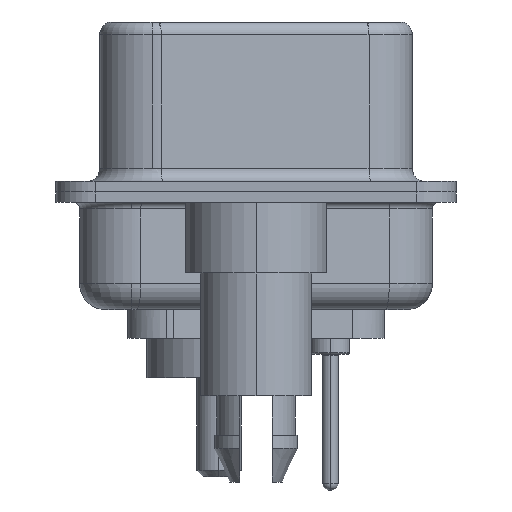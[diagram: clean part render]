
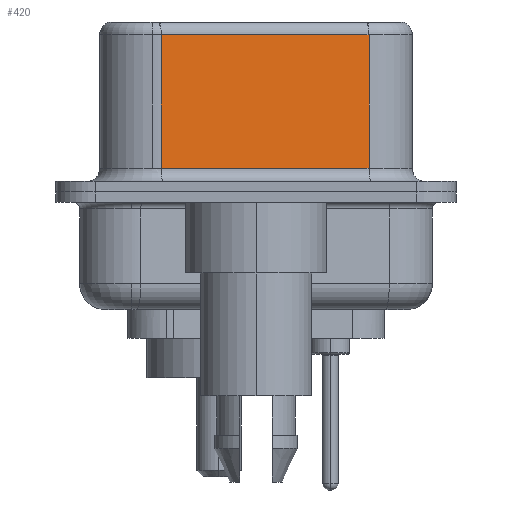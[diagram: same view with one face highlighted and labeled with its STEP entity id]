
A CAD part, left-side view. The second image highlights one B-rep face of the part: STEP entity #420.
In plain terms, the highlighted planar face has unit normal (-0.985, -0.174, 0).
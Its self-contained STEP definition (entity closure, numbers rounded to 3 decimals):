
#354 = PLANE ( 'NONE',  #21658 ) ;
#420 = ADVANCED_FACE ( 'NONE', ( #16871 ), #354, .F. ) ;
#1713 = VECTOR ( 'NONE', #21251, 1000. ) ;
#2260 = LINE ( 'NONE', #19577, #1713 ) ;
#2346 = VERTEX_POINT ( 'NONE', #6088 ) ;
#2419 = ORIENTED_EDGE ( 'NONE', *, *, #6296, .T. ) ;
#3163 = EDGE_LOOP ( 'NONE', ( #19923, #2419, #15302, #13762 ) ) ;
#3882 = DIRECTION ( 'NONE',  ( -0.174, 0.985, 0. ) ) ;
#4128 = CARTESIAN_POINT ( 'NONE',  ( 5.132, -4.322, 6.02 ) ) ;
#5108 = CARTESIAN_POINT ( 'NONE',  ( 5.132, -4.322, 6.52 ) ) ;
#5414 = EDGE_CURVE ( 'NONE', #2346, #11596, #9082, .T. ) ;
#5584 = CARTESIAN_POINT ( 'NONE',  ( 5.132, -4.322, 6.52 ) ) ;
#6088 = CARTESIAN_POINT ( 'NONE',  ( 3.73, 3.628, 6.02 ) ) ;
#6296 = EDGE_CURVE ( 'NONE', #20462, #2346, #14081, .T. ) ;
#6843 = DIRECTION ( 'NONE',  ( 0., 0., -1. ) ) ;
#8311 = EDGE_CURVE ( 'NONE', #20462, #18984, #15265, .T. ) ;
#8675 = DIRECTION ( 'NONE',  ( 0., 0., -1. ) ) ;
#9082 = LINE ( 'NONE', #20441, #13053 ) ;
#9578 = VECTOR ( 'NONE', #21714, 1000. ) ;
#9673 = EDGE_CURVE ( 'NONE', #11596, #18984, #2260, .T. ) ;
#10810 = VECTOR ( 'NONE', #6843, 1000. ) ;
#11596 = VERTEX_POINT ( 'NONE', #19435 ) ;
#13053 = VECTOR ( 'NONE', #8675, 1000. ) ;
#13762 = ORIENTED_EDGE ( 'NONE', *, *, #9673, .T. ) ;
#14081 = LINE ( 'NONE', #20017, #9578 ) ;
#14198 = DIRECTION ( 'NONE',  ( 0.985, 0.174, 0. ) ) ;
#14260 = CARTESIAN_POINT ( 'NONE',  ( 5.132, -4.322, 0.9 ) ) ;
#15265 = LINE ( 'NONE', #5108, #10810 ) ;
#15302 = ORIENTED_EDGE ( 'NONE', *, *, #5414, .T. ) ;
#16871 = FACE_OUTER_BOUND ( 'NONE', #3163, .T. ) ;
#18984 = VERTEX_POINT ( 'NONE', #14260 ) ;
#19435 = CARTESIAN_POINT ( 'NONE',  ( 3.73, 3.628, 0.9 ) ) ;
#19577 = CARTESIAN_POINT ( 'NONE',  ( 5.132, -4.322, 0.9 ) ) ;
#19923 = ORIENTED_EDGE ( 'NONE', *, *, #8311, .F. ) ;
#20017 = CARTESIAN_POINT ( 'NONE',  ( 5.132, -4.322, 6.02 ) ) ;
#20441 = CARTESIAN_POINT ( 'NONE',  ( 3.73, 3.628, 6.52 ) ) ;
#20462 = VERTEX_POINT ( 'NONE', #4128 ) ;
#21251 = DIRECTION ( 'NONE',  ( 0.174, -0.985, 0. ) ) ;
#21658 = AXIS2_PLACEMENT_3D ( 'NONE', #5584, #14198, #3882 ) ;
#21714 = DIRECTION ( 'NONE',  ( -0.174, 0.985, 0. ) ) ;
